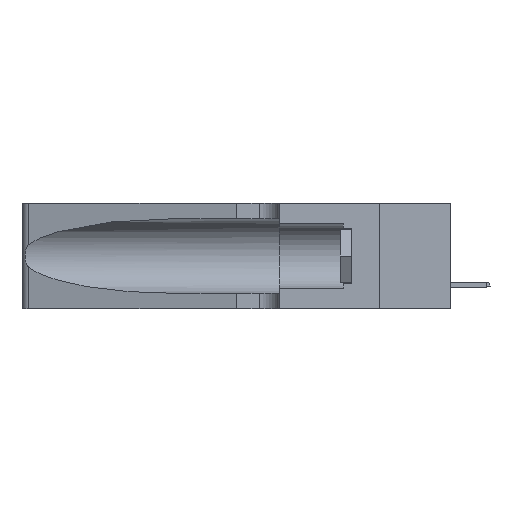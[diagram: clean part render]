
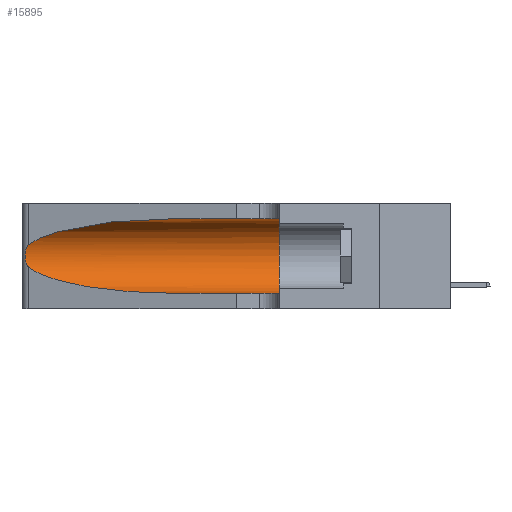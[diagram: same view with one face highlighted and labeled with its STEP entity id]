
A CAD part, left-side view. The second image highlights one B-rep face of the part: STEP entity #15895.
In plain terms, the highlighted cylindrical face has radius 3.308 mm (diameter 6.617 mm), a partial arc.
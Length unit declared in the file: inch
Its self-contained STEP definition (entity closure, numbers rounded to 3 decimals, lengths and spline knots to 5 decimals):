
#305 = EDGE_LOOP ( 'NONE', ( #11220, #9004, #21585, #19183, #9188, #11572 ) ) ;
#310 = CYLINDRICAL_SURFACE ( 'NONE', #11975, 0.13025 ) ;
#568 = CARTESIAN_POINT ( 'NONE',  ( 0.1305, 1.61858, 0.185 ) ) ;
#719 = CARTESIAN_POINT ( 'NONE',  ( 0.1305, 1.61858, 0.31525 ) ) ;
#774 = CARTESIAN_POINT ( 'NONE',  ( 0.1305, 0.72297, 0.31525 ) ) ;
#1124 = CARTESIAN_POINT ( 'NONE',  ( 0.26075, 1.23896, 0.178 ) ) ;
#2621 = LINE ( 'NONE', #12796, #2764 ) ;
#2676 = EDGE_CURVE ( 'NONE', #25686, #3451, #4983, .T. ) ;
#2764 = VECTOR ( 'NONE', #15062, 39.37008 ) ;
#3097 = CARTESIAN_POINT ( 'NONE',  ( 0.1305, 0.72297, 0.05475 ) ) ;
#3119 = CARTESIAN_POINT ( 'NONE',  ( 0.25487, 1.22718, 0.14631 ) ) ;
#3451 = VERTEX_POINT ( 'NONE', #14966 ) ;
#4151 = DIRECTION ( 'NONE',  ( 0., 0., 1. ) ) ;
#4970 = CARTESIAN_POINT ( 'NONE',  ( 0.18966, 0.96281, 0.05475 ) ) ;
#4983 = LINE ( 'NONE', #719, #6428 ) ;
#5382 = CARTESIAN_POINT ( 'NONE',  ( 0.25787, 1.23484, 0.2124 ) ) ;
#5517 = CARTESIAN_POINT ( 'NONE',  ( 0.25487, 1.22718, 0.22369 ) ) ;
#5686 = VERTEX_POINT ( 'NONE', #25864 ) ;
#6352 = VERTEX_POINT ( 'NONE', #24969 ) ;
#6428 = VECTOR ( 'NONE', #16783, 39.37008 ) ;
#7109 = CARTESIAN_POINT ( 'NONE',  ( 0.26018, 1.23835, 0.19895 ) ) ;
#7413 = EDGE_CURVE ( 'NONE', #5686, #19094, #19436, .T. ) ;
#7512 = CARTESIAN_POINT ( 'NONE',  ( 0.25789, 1.23486, 0.15765 ) ) ;
#8548 = EDGE_CURVE ( 'NONE', #19094, #19443, #2621, .T. ) ;
#9004 = ORIENTED_EDGE ( 'NONE', *, *, #10330, .T. ) ;
#9143 = CARTESIAN_POINT ( 'NONE',  ( 0.26017, 1.23833, 0.17102 ) ) ;
#9188 = ORIENTED_EDGE ( 'NONE', *, *, #25142, .F. ) ;
#9456 = CARTESIAN_POINT ( 'NONE',  ( 0.25487, 1.22718, 0.22369 ) ) ;
#10330 = EDGE_CURVE ( 'NONE', #6352, #5686, #12956, .T. ) ;
#10402 = CIRCLE ( 'NONE', #25356, 0.13025 ) ;
#11220 = ORIENTED_EDGE ( 'NONE', *, *, #16217, .T. ) ;
#11572 = ORIENTED_EDGE ( 'NONE', *, *, #2676, .F. ) ;
#11975 = AXIS2_PLACEMENT_3D ( 'NONE', #568, #16762, #22887 ) ;
#12796 = CARTESIAN_POINT ( 'NONE',  ( 0.1305, 1.61858, 0.05475 ) ) ;
#12956 = B_SPLINE_CURVE_WITH_KNOTS ( 'NONE', 3,
 ( #5517, #25858, #21822, #5382, #13564, #7109, #17313, #1124, #9143, #21688, #7512, #19580, #15697, #3119 ),
 .UNSPECIFIED., .F., .F.,
 ( 4, 2, 2, 2, 2, 2, 4 ),
 ( 0., 0.00027, 0.00053, 0.00107, 0.0016, 0.00187, 0.00214 ),
 .UNSPECIFIED. ) ;
#13564 = CARTESIAN_POINT ( 'NONE',  ( 0.25854, 1.2359, 0.20912 ) ) ;
#14460 = DIRECTION ( 'NONE',  ( 0., 1., 0. ) ) ;
#14616 = FACE_OUTER_BOUND ( 'NONE', #305, .T. ) ;
#14966 = CARTESIAN_POINT ( 'NONE',  ( 0.1305, 0.35, 0.31525 ) ) ;
#15062 = DIRECTION ( 'NONE',  ( 0., -1., 0. ) ) ;
#15234 = CARTESIAN_POINT ( 'NONE',  ( 0.2373, 1.15595, 0.28018 ) ) ;
#15367 = CARTESIAN_POINT ( 'NONE',  ( 0.1305, 0.72297, 0.31525 ) ) ;
#15697 = CARTESIAN_POINT ( 'NONE',  ( 0.25555, 1.22993, 0.14849 ) ) ;
#15895 = ADVANCED_FACE ( 'NONE', ( #14616 ), #310, .F. ) ;
#16217 = EDGE_CURVE ( 'NONE', #25686, #6352, #22150, .T. ) ;
#16762 = DIRECTION ( 'NONE',  ( 0., -1., 0. ) ) ;
#16783 = DIRECTION ( 'NONE',  ( 0., -1., 0. ) ) ;
#17313 = CARTESIAN_POINT ( 'NONE',  ( 0.26075, 1.23896, 0.19203 ) ) ;
#18966 = CARTESIAN_POINT ( 'NONE',  ( 0.1305, 0.72297, 0.05475 ) ) ;
#19094 = VERTEX_POINT ( 'NONE', #18966 ) ;
#19183 = ORIENTED_EDGE ( 'NONE', *, *, #8548, .T. ) ;
#19436 =( BOUNDED_CURVE ( )  B_SPLINE_CURVE ( 3, ( #23301, #25040, #4970, #3097 ),
 .UNSPECIFIED., .F., .F. ) 
 B_SPLINE_CURVE_WITH_KNOTS ( ( 4, 4 ),
 ( 3.44316, 4.71239 ),
 .UNSPECIFIED. ) 
 CURVE ( )  GEOMETRIC_REPRESENTATION_ITEM ( )  RATIONAL_B_SPLINE_CURVE ( ( 1., 0.87, 0.87, 1. ) ) 
 REPRESENTATION_ITEM ( '' )  );
#19443 = VERTEX_POINT ( 'NONE', #20266 ) ;
#19580 = CARTESIAN_POINT ( 'NONE',  ( 0.25639, 1.23186, 0.15144 ) ) ;
#19631 = CARTESIAN_POINT ( 'NONE',  ( 0.18966, 0.96281, 0.31525 ) ) ;
#20073 = CARTESIAN_POINT ( 'NONE',  ( 0.1305, 0.35, 0.185 ) ) ;
#20266 = CARTESIAN_POINT ( 'NONE',  ( 0.1305, 0.35, 0.05475 ) ) ;
#21585 = ORIENTED_EDGE ( 'NONE', *, *, #7413, .T. ) ;
#21688 = CARTESIAN_POINT ( 'NONE',  ( 0.25856, 1.23593, 0.16098 ) ) ;
#21822 = CARTESIAN_POINT ( 'NONE',  ( 0.25639, 1.23184, 0.21858 ) ) ;
#22150 =( BOUNDED_CURVE ( )  B_SPLINE_CURVE ( 3, ( #15367, #19631, #15234, #9456 ),
 .UNSPECIFIED., .F., .F. ) 
 B_SPLINE_CURVE_WITH_KNOTS ( ( 4, 4 ),
 ( 1.5708, 2.84003 ),
 .UNSPECIFIED. ) 
 CURVE ( )  GEOMETRIC_REPRESENTATION_ITEM ( )  RATIONAL_B_SPLINE_CURVE ( ( 1., 0.87, 0.87, 1. ) ) 
 REPRESENTATION_ITEM ( '' )  );
#22887 = DIRECTION ( 'NONE',  ( 0., 0., -1. ) ) ;
#23301 = CARTESIAN_POINT ( 'NONE',  ( 0.25487, 1.22718, 0.14631 ) ) ;
#24969 = CARTESIAN_POINT ( 'NONE',  ( 0.25487, 1.22718, 0.22369 ) ) ;
#25040 = CARTESIAN_POINT ( 'NONE',  ( 0.2373, 1.15595, 0.08982 ) ) ;
#25142 = EDGE_CURVE ( 'NONE', #3451, #19443, #10402, .T. ) ;
#25356 = AXIS2_PLACEMENT_3D ( 'NONE', #20073, #14460, #4151 ) ;
#25686 = VERTEX_POINT ( 'NONE', #774 ) ;
#25858 = CARTESIAN_POINT ( 'NONE',  ( 0.25555, 1.22994, 0.2215 ) ) ;
#25864 = CARTESIAN_POINT ( 'NONE',  ( 0.25487, 1.22718, 0.14631 ) ) ;
